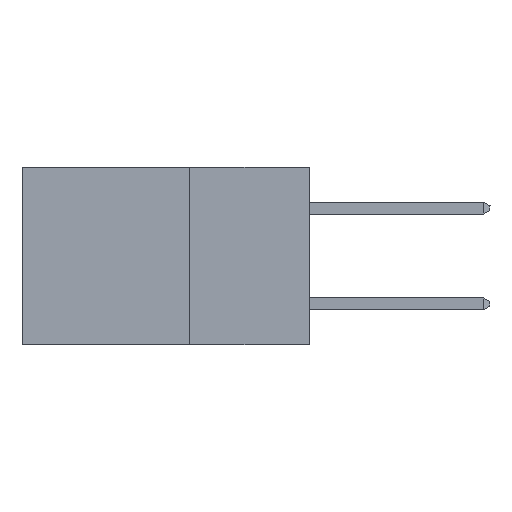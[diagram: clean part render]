
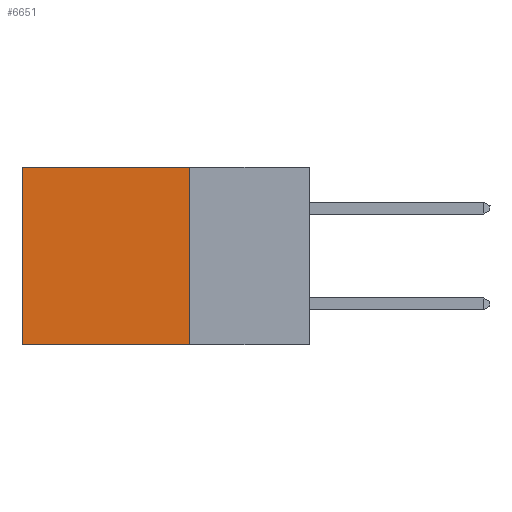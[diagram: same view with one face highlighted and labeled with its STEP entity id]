
A CAD part, left-side view. The second image highlights one B-rep face of the part: STEP entity #6651.
In plain terms, the highlighted planar face has unit normal (-1, 0, 0).
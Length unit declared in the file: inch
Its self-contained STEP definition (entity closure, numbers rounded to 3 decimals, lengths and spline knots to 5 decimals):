
#1364 = DIRECTION ( 'NONE',  ( 0., 0., -1. ) ) ;
#1441 = CARTESIAN_POINT ( 'NONE',  ( 0.2875, 0.6, -0.37 ) ) ;
#1643 = CARTESIAN_POINT ( 'NONE',  ( 0.2875, 0.25, 0. ) ) ;
#1903 = CARTESIAN_POINT ( 'NONE',  ( 0.2875, 0.6, 0. ) ) ;
#2191 = CARTESIAN_POINT ( 'NONE',  ( 0.2875, 0.25, 0. ) ) ;
#2691 = VECTOR ( 'NONE', #9721, 39.37008 ) ;
#2827 = DIRECTION ( 'NONE',  ( 0., 0., -1. ) ) ;
#3440 = VECTOR ( 'NONE', #14817, 39.37008 ) ;
#3880 = LINE ( 'NONE', #1903, #3440 ) ;
#3927 = ORIENTED_EDGE ( 'NONE', *, *, #11149, .T. ) ;
#4017 = ORIENTED_EDGE ( 'NONE', *, *, #11566, .F. ) ;
#4025 = CARTESIAN_POINT ( 'NONE',  ( 0.2875, 0.25, -0.37 ) ) ;
#4123 = ORIENTED_EDGE ( 'NONE', *, *, #9265, .F. ) ;
#4137 = ORIENTED_EDGE ( 'NONE', *, *, #8116, .T. ) ;
#4777 = CARTESIAN_POINT ( 'NONE',  ( 0.2875, 0.25, -0.37 ) ) ;
#5342 = DIRECTION ( 'NONE',  ( 0., 1., 0. ) ) ;
#6124 = VERTEX_POINT ( 'NONE', #1441 ) ;
#6211 = LINE ( 'NONE', #14803, #2691 ) ;
#6254 = VERTEX_POINT ( 'NONE', #6994 ) ;
#6367 = LINE ( 'NONE', #1643, #12374 ) ;
#6651 = ADVANCED_FACE ( 'NONE', ( #12610 ), #12959, .F. ) ;
#6994 = CARTESIAN_POINT ( 'NONE',  ( 0.2875, 0.6, 0. ) ) ;
#8116 = EDGE_CURVE ( 'NONE', #9567, #6254, #6211, .T. ) ;
#8191 = VERTEX_POINT ( 'NONE', #4777 ) ;
#9134 = DIRECTION ( 'NONE',  ( 1., 0., 0. ) ) ;
#9265 = EDGE_CURVE ( 'NONE', #9567, #8191, #6367, .T. ) ;
#9567 = VERTEX_POINT ( 'NONE', #2191 ) ;
#9721 = DIRECTION ( 'NONE',  ( 0., 1., 0. ) ) ;
#11149 = EDGE_CURVE ( 'NONE', #6254, #6124, #3880, .T. ) ;
#11476 = LINE ( 'NONE', #4025, #14463 ) ;
#11566 = EDGE_CURVE ( 'NONE', #8191, #6124, #11476, .T. ) ;
#12374 = VECTOR ( 'NONE', #2827, 39.37008 ) ;
#12610 = FACE_OUTER_BOUND ( 'NONE', #12995, .T. ) ;
#12959 = PLANE ( 'NONE',  #13817 ) ;
#12995 = EDGE_LOOP ( 'NONE', ( #3927, #4017, #4123, #4137 ) ) ;
#13817 = AXIS2_PLACEMENT_3D ( 'NONE', #15507, #9134, #1364 ) ;
#14463 = VECTOR ( 'NONE', #5342, 39.37008 ) ;
#14803 = CARTESIAN_POINT ( 'NONE',  ( 0.2875, 0.25, 0. ) ) ;
#14817 = DIRECTION ( 'NONE',  ( 0., 0., -1. ) ) ;
#15507 = CARTESIAN_POINT ( 'NONE',  ( 0.2875, 0.25, 0. ) ) ;
